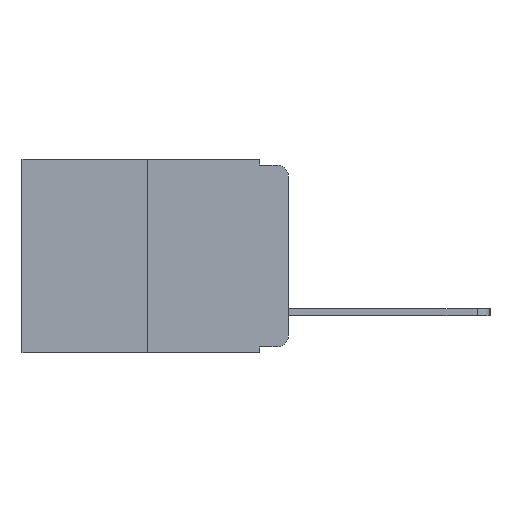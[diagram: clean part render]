
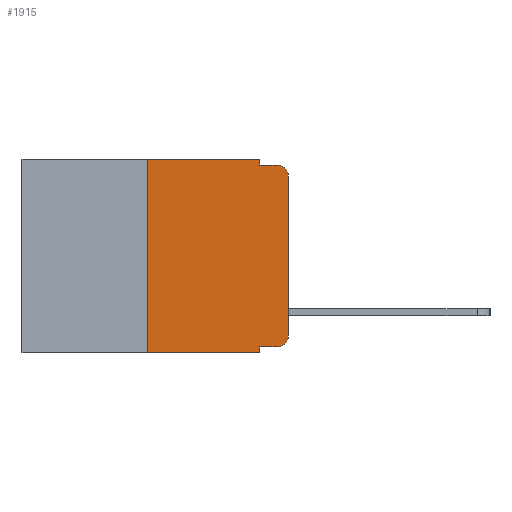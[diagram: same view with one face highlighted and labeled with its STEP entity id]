
A CAD part, left-side view. The second image highlights one B-rep face of the part: STEP entity #1915.
In plain terms, the highlighted planar face has unit normal (-1, 0, 0).
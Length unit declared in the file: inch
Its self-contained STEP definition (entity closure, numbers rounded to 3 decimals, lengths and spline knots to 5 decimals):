
#63 = AXIS2_PLACEMENT_3D ( 'NONE', #2053, #121, #8705 ) ;
#86 = DIRECTION ( 'NONE',  ( 0., 0., -1. ) ) ;
#110 = CARTESIAN_POINT ( 'NONE',  ( 0., 0.02, -0.313 ) ) ;
#121 = DIRECTION ( 'NONE',  ( 1., 0., 0. ) ) ;
#294 = CARTESIAN_POINT ( 'NONE',  ( 0., 0., 0. ) ) ;
#751 = FACE_OUTER_BOUND ( 'NONE', #5134, .T. ) ;
#812 = EDGE_CURVE ( 'NONE', #20701, #6580, #16660, .T. ) ;
#1090 = VERTEX_POINT ( 'NONE', #15030 ) ;
#1453 = PLANE ( 'NONE',  #63 ) ;
#1787 = DIRECTION ( 'NONE',  ( 0., 0., -1. ) ) ;
#1915 = ADVANCED_FACE ( 'NONE', ( #751 ), #1453, .F. ) ;
#2053 = CARTESIAN_POINT ( 'NONE',  ( 0., 0.473, 0. ) ) ;
#2532 = ORIENTED_EDGE ( 'NONE', *, *, #17380, .T. ) ;
#3001 = EDGE_CURVE ( 'NONE', #6580, #14404, #17561, .T. ) ;
#3721 = CIRCLE ( 'NONE', #9213, 0.02 ) ;
#3737 = CARTESIAN_POINT ( 'NONE',  ( 0., 0., -0.313 ) ) ;
#3813 = AXIS2_PLACEMENT_3D ( 'NONE', #12363, #14475, #10481 ) ;
#3926 = CARTESIAN_POINT ( 'NONE',  ( 0., 0.473, 0. ) ) ;
#4048 = ORIENTED_EDGE ( 'NONE', *, *, #3001, .F. ) ;
#4076 = EDGE_CURVE ( 'NONE', #1090, #14404, #9711, .T. ) ;
#4089 = CARTESIAN_POINT ( 'NONE',  ( 0., 0.25, -0.343 ) ) ;
#4223 = LINE ( 'NONE', #7918, #7948 ) ;
#4261 = VECTOR ( 'NONE', #14293, 39.37008 ) ;
#5134 = EDGE_LOOP ( 'NONE', ( #9298, #13055, #4048, #5562, #13070, #8292, #20055, #11571, #2532, #14319 ) ) ;
#5148 = EDGE_CURVE ( 'NONE', #7890, #1090, #10914, .T. ) ;
#5191 = LINE ( 'NONE', #15792, #8420 ) ;
#5427 = CARTESIAN_POINT ( 'NONE',  ( 0., 0.051, -0.343 ) ) ;
#5562 = ORIENTED_EDGE ( 'NONE', *, *, #812, .F. ) ;
#5813 = DIRECTION ( 'NONE',  ( 0., 0., 1. ) ) ;
#6580 = VERTEX_POINT ( 'NONE', #17757 ) ;
#7890 = VERTEX_POINT ( 'NONE', #3737 ) ;
#7918 = CARTESIAN_POINT ( 'NONE',  ( 0., 0.051, -0.333 ) ) ;
#7948 = VECTOR ( 'NONE', #17351, 39.37008 ) ;
#8021 = VERTEX_POINT ( 'NONE', #4089 ) ;
#8292 = ORIENTED_EDGE ( 'NONE', *, *, #20514, .F. ) ;
#8420 = VECTOR ( 'NONE', #17418, 39.37008 ) ;
#8615 = VECTOR ( 'NONE', #5813, 39.37008 ) ;
#8705 = DIRECTION ( 'NONE',  ( 0., 0., -1. ) ) ;
#8859 = DIRECTION ( 'NONE',  ( 0., 0., 1. ) ) ;
#9213 = AXIS2_PLACEMENT_3D ( 'NONE', #110, #11415, #1787 ) ;
#9298 = ORIENTED_EDGE ( 'NONE', *, *, #5148, .T. ) ;
#9316 = CARTESIAN_POINT ( 'NONE',  ( 0., 0.25, 0. ) ) ;
#9711 = CIRCLE ( 'NONE', #3813, 0.02 ) ;
#10098 = EDGE_CURVE ( 'NONE', #8021, #14079, #15788, .T. ) ;
#10378 = EDGE_CURVE ( 'NONE', #20632, #20701, #17806, .T. ) ;
#10481 = DIRECTION ( 'NONE',  ( 0., 0., -1. ) ) ;
#10914 = LINE ( 'NONE', #294, #13151 ) ;
#11012 = VECTOR ( 'NONE', #16069, 39.37008 ) ;
#11415 = DIRECTION ( 'NONE',  ( -1., 0., 0. ) ) ;
#11571 = ORIENTED_EDGE ( 'NONE', *, *, #19490, .F. ) ;
#11798 = CARTESIAN_POINT ( 'NONE',  ( 0., 0.051, 0. ) ) ;
#12069 = VERTEX_POINT ( 'NONE', #20465 ) ;
#12363 = CARTESIAN_POINT ( 'NONE',  ( 0., 0.02, -0.03 ) ) ;
#12404 = VERTEX_POINT ( 'NONE', #13335 ) ;
#13055 = ORIENTED_EDGE ( 'NONE', *, *, #4076, .T. ) ;
#13070 = ORIENTED_EDGE ( 'NONE', *, *, #10378, .F. ) ;
#13108 = CARTESIAN_POINT ( 'NONE',  ( 0., 0.02, -0.01 ) ) ;
#13151 = VECTOR ( 'NONE', #8859, 39.37008 ) ;
#13335 = CARTESIAN_POINT ( 'NONE',  ( 0., 0.051, -0.333 ) ) ;
#13497 = VECTOR ( 'NONE', #19930, 39.37008 ) ;
#14079 = VERTEX_POINT ( 'NONE', #5427 ) ;
#14268 = CARTESIAN_POINT ( 'NONE',  ( 0., 0.051, -0.01 ) ) ;
#14293 = DIRECTION ( 'NONE',  ( 0., -1., 0. ) ) ;
#14319 = ORIENTED_EDGE ( 'NONE', *, *, #16310, .T. ) ;
#14404 = VERTEX_POINT ( 'NONE', #13108 ) ;
#14475 = DIRECTION ( 'NONE',  ( -1., 0., 0. ) ) ;
#15030 = CARTESIAN_POINT ( 'NONE',  ( 0., 0., -0.03 ) ) ;
#15430 = CARTESIAN_POINT ( 'NONE',  ( 0., 0.25, 0. ) ) ;
#15788 = LINE ( 'NONE', #19211, #11012 ) ;
#15792 = CARTESIAN_POINT ( 'NONE',  ( 0., 0.051, 0. ) ) ;
#15927 = CARTESIAN_POINT ( 'NONE',  ( 0., 0.051, 0. ) ) ;
#16069 = DIRECTION ( 'NONE',  ( 0., -1., 0. ) ) ;
#16310 = EDGE_CURVE ( 'NONE', #12069, #7890, #3721, .T. ) ;
#16660 = LINE ( 'NONE', #11798, #20338 ) ;
#17185 = LINE ( 'NONE', #15430, #8615 ) ;
#17351 = DIRECTION ( 'NONE',  ( 0., -1., 0. ) ) ;
#17380 = EDGE_CURVE ( 'NONE', #12404, #12069, #4223, .T. ) ;
#17418 = DIRECTION ( 'NONE',  ( 0., 0., -1. ) ) ;
#17561 = LINE ( 'NONE', #14268, #4261 ) ;
#17757 = CARTESIAN_POINT ( 'NONE',  ( 0., 0.051, -0.01 ) ) ;
#17806 = LINE ( 'NONE', #3926, #13497 ) ;
#19211 = CARTESIAN_POINT ( 'NONE',  ( 0., 0.473, -0.343 ) ) ;
#19490 = EDGE_CURVE ( 'NONE', #12404, #14079, #5191, .T. ) ;
#19930 = DIRECTION ( 'NONE',  ( 0., -1., 0. ) ) ;
#20055 = ORIENTED_EDGE ( 'NONE', *, *, #10098, .T. ) ;
#20338 = VECTOR ( 'NONE', #86, 39.37008 ) ;
#20465 = CARTESIAN_POINT ( 'NONE',  ( 0., 0.02, -0.333 ) ) ;
#20514 = EDGE_CURVE ( 'NONE', #8021, #20632, #17185, .T. ) ;
#20632 = VERTEX_POINT ( 'NONE', #9316 ) ;
#20701 = VERTEX_POINT ( 'NONE', #15927 ) ;
